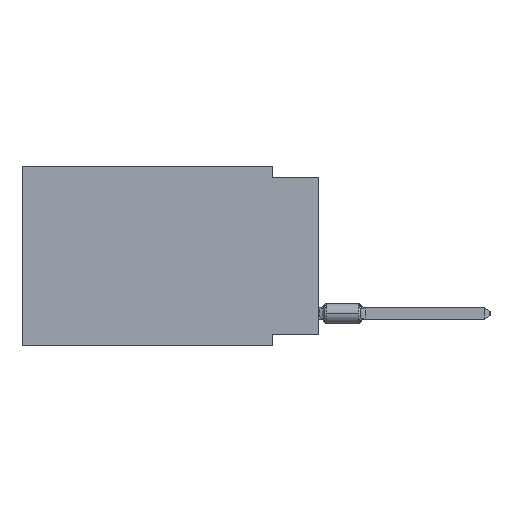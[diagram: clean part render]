
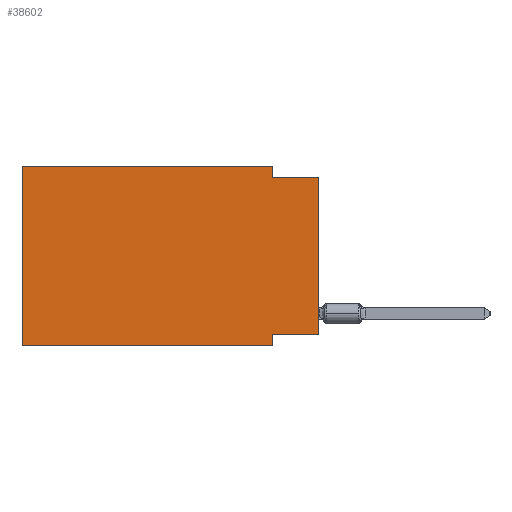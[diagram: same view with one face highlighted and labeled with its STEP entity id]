
A CAD part, left-side view. The second image highlights one B-rep face of the part: STEP entity #38602.
In plain terms, the highlighted planar face has unit normal (-1, 0, 0).
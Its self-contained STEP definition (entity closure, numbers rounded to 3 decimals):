
#704 = LINE ( 'NONE', #19741, #7767 ) ;
#2058 = ORIENTED_EDGE ( 'NONE', *, *, #26590, .F. ) ;
#3554 = CARTESIAN_POINT ( 'NONE',  ( 0., 0., -0.635 ) ) ;
#4859 = CARTESIAN_POINT ( 'NONE',  ( 0., 2.54, -0.635 ) ) ;
#6107 = VERTEX_POINT ( 'NONE', #4859 ) ;
#7767 = VECTOR ( 'NONE', #38472, 1000. ) ;
#8721 = CARTESIAN_POINT ( 'NONE',  ( 0., 0., -9.271 ) ) ;
#9305 = ORIENTED_EDGE ( 'NONE', *, *, #57142, .T. ) ;
#9860 = LINE ( 'NONE', #28625, #17956 ) ;
#9966 = CARTESIAN_POINT ( 'NONE',  ( 0., 2.54, -9.906 ) ) ;
#11648 = CARTESIAN_POINT ( 'NONE',  ( 0., 16.383, 0. ) ) ;
#14214 = DIRECTION ( 'NONE',  ( 0., 0., -1. ) ) ;
#16709 = LINE ( 'NONE', #44650, #59008 ) ;
#17956 = VECTOR ( 'NONE', #33830, 1000. ) ;
#19270 = EDGE_CURVE ( 'NONE', #6107, #26261, #704, .T. ) ;
#19741 = CARTESIAN_POINT ( 'NONE',  ( 0., 0., -0.635 ) ) ;
#19888 = DIRECTION ( 'NONE',  ( 0., 0., 1. ) ) ;
#20103 = DIRECTION ( 'NONE',  ( 0., -1., 0. ) ) ;
#21523 = VECTOR ( 'NONE', #19888, 1000. ) ;
#23227 = CARTESIAN_POINT ( 'NONE',  ( 0., 2.54, -9.271 ) ) ;
#23590 = CARTESIAN_POINT ( 'NONE',  ( 0., 2.54, 0. ) ) ;
#24037 = EDGE_CURVE ( 'NONE', #37368, #45526, #42311, .T. ) ;
#26261 = VERTEX_POINT ( 'NONE', #3554 ) ;
#26347 = ORIENTED_EDGE ( 'NONE', *, *, #56625, .T. ) ;
#26590 = EDGE_CURVE ( 'NONE', #47318, #54810, #16709, .T. ) ;
#27344 = VECTOR ( 'NONE', #35759, 1000. ) ;
#27927 = DIRECTION ( 'NONE',  ( 0., -1., 0. ) ) ;
#27958 = ORIENTED_EDGE ( 'NONE', *, *, #24037, .F. ) ;
#28144 = EDGE_CURVE ( 'NONE', #45526, #42938, #46831, .T. ) ;
#28625 = CARTESIAN_POINT ( 'NONE',  ( 0., 0., -9.271 ) ) ;
#29751 = VECTOR ( 'NONE', #20103, 1000. ) ;
#30444 = VERTEX_POINT ( 'NONE', #8721 ) ;
#31102 = EDGE_LOOP ( 'NONE', ( #26347, #36993, #40851, #36298, #27958, #9305, #2058, #45134 ) ) ;
#32055 = DIRECTION ( 'NONE',  ( 0., 0., -1. ) ) ;
#33753 = CARTESIAN_POINT ( 'NONE',  ( 0., 16.383, -9.906 ) ) ;
#33830 = DIRECTION ( 'NONE',  ( 0., 1., 0. ) ) ;
#35444 = DIRECTION ( 'NONE',  ( 0., 0., -1. ) ) ;
#35759 = DIRECTION ( 'NONE',  ( 0., 0., 1. ) ) ;
#36298 = ORIENTED_EDGE ( 'NONE', *, *, #28144, .F. ) ;
#36993 = ORIENTED_EDGE ( 'NONE', *, *, #19270, .F. ) ;
#37368 = VERTEX_POINT ( 'NONE', #39448 ) ;
#37431 = LINE ( 'NONE', #33753, #40155 ) ;
#37575 = CARTESIAN_POINT ( 'NONE',  ( 0., 2.54, 0. ) ) ;
#38472 = DIRECTION ( 'NONE',  ( 0., -1., 0. ) ) ;
#38602 = ADVANCED_FACE ( 'NONE', ( #45859 ), #56020, .F. ) ;
#39334 = VECTOR ( 'NONE', #14214, 1000. ) ;
#39448 = CARTESIAN_POINT ( 'NONE',  ( 0., 16.383, -9.906 ) ) ;
#40155 = VECTOR ( 'NONE', #27927, 1000. ) ;
#40368 = EDGE_CURVE ( 'NONE', #30444, #47318, #9860, .T. ) ;
#40384 = LINE ( 'NONE', #59106, #27344 ) ;
#40851 = ORIENTED_EDGE ( 'NONE', *, *, #46658, .F. ) ;
#41868 = LINE ( 'NONE', #37575, #39334 ) ;
#42311 = LINE ( 'NONE', #42917, #21523 ) ;
#42391 = AXIS2_PLACEMENT_3D ( 'NONE', #51411, #60307, #32055 ) ;
#42840 = CARTESIAN_POINT ( 'NONE',  ( 0., 16.383, 0. ) ) ;
#42917 = CARTESIAN_POINT ( 'NONE',  ( 0., 16.383, 0. ) ) ;
#42938 = VERTEX_POINT ( 'NONE', #23590 ) ;
#44650 = CARTESIAN_POINT ( 'NONE',  ( 0., 2.54, -9.906 ) ) ;
#45134 = ORIENTED_EDGE ( 'NONE', *, *, #40368, .F. ) ;
#45526 = VERTEX_POINT ( 'NONE', #11648 ) ;
#45859 = FACE_OUTER_BOUND ( 'NONE', #31102, .T. ) ;
#46658 = EDGE_CURVE ( 'NONE', #42938, #6107, #41868, .T. ) ;
#46831 = LINE ( 'NONE', #42840, #29751 ) ;
#47318 = VERTEX_POINT ( 'NONE', #23227 ) ;
#51411 = CARTESIAN_POINT ( 'NONE',  ( 0., 16.383, 0. ) ) ;
#54810 = VERTEX_POINT ( 'NONE', #9966 ) ;
#56020 = PLANE ( 'NONE',  #42391 ) ;
#56625 = EDGE_CURVE ( 'NONE', #30444, #26261, #40384, .T. ) ;
#57142 = EDGE_CURVE ( 'NONE', #37368, #54810, #37431, .T. ) ;
#59008 = VECTOR ( 'NONE', #35444, 1000. ) ;
#59106 = CARTESIAN_POINT ( 'NONE',  ( 0., 0., 0. ) ) ;
#60307 = DIRECTION ( 'NONE',  ( 1., 0., 0. ) ) ;
